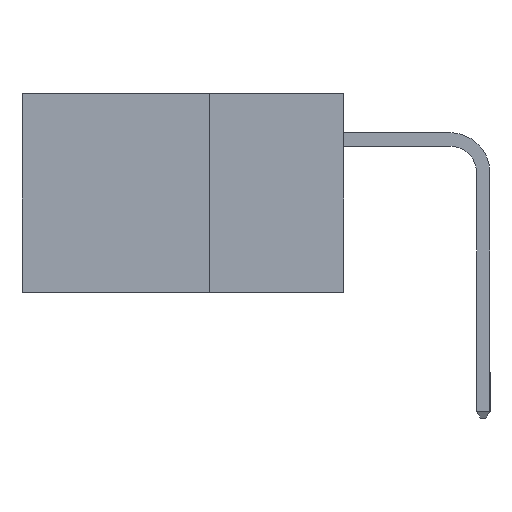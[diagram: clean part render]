
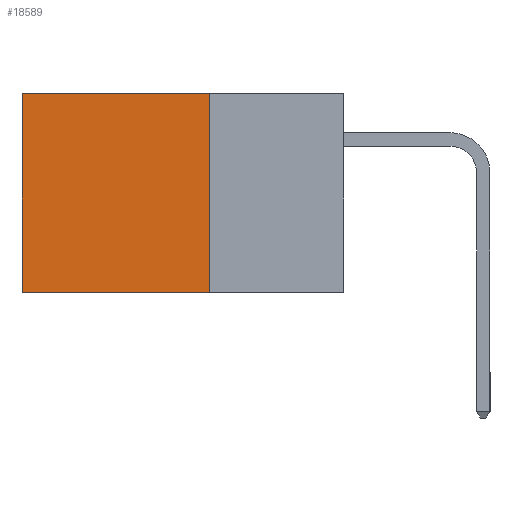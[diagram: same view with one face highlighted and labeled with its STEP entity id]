
A CAD part, left-side view. The second image highlights one B-rep face of the part: STEP entity #18589.
In plain terms, the highlighted planar face has unit normal (-1, 0, 0).
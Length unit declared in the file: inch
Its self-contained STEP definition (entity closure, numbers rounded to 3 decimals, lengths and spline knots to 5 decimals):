
#692 = DIRECTION ( 'NONE',  ( 1., 0., 0. ) ) ;
#1110 = VECTOR ( 'NONE', #4882, 39.37008 ) ;
#3337 = EDGE_LOOP ( 'NONE', ( #21907, #8122, #11441, #19299 ) ) ;
#3561 = EDGE_CURVE ( 'NONE', #12303, #6107, #20662, .T. ) ;
#4045 = CARTESIAN_POINT ( 'NONE',  ( 0.298, 0.25, -0.37 ) ) ;
#4882 = DIRECTION ( 'NONE',  ( 0., 0., -1. ) ) ;
#5588 = VECTOR ( 'NONE', #7385, 39.37008 ) ;
#5872 = AXIS2_PLACEMENT_3D ( 'NONE', #7417, #692, #7344 ) ;
#6041 = DIRECTION ( 'NONE',  ( 0., 1., 0. ) ) ;
#6107 = VERTEX_POINT ( 'NONE', #12417 ) ;
#6580 = VERTEX_POINT ( 'NONE', #14096 ) ;
#6591 = CARTESIAN_POINT ( 'NONE',  ( 0.298, 0.6, 0. ) ) ;
#7272 = FACE_OUTER_BOUND ( 'NONE', #3337, .T. ) ;
#7344 = DIRECTION ( 'NONE',  ( 0., 0., -1. ) ) ;
#7385 = DIRECTION ( 'NONE',  ( 0., 1., 0. ) ) ;
#7417 = CARTESIAN_POINT ( 'NONE',  ( 0.298, 0.25, 0. ) ) ;
#8122 = ORIENTED_EDGE ( 'NONE', *, *, #16086, .F. ) ;
#10761 = EDGE_CURVE ( 'NONE', #16242, #6580, #15560, .T. ) ;
#11339 = DIRECTION ( 'NONE',  ( 0., 0., -1. ) ) ;
#11441 = ORIENTED_EDGE ( 'NONE', *, *, #3561, .F. ) ;
#12303 = VERTEX_POINT ( 'NONE', #14629 ) ;
#12417 = CARTESIAN_POINT ( 'NONE',  ( 0.298, 0.25, -0.37 ) ) ;
#12716 = PLANE ( 'NONE',  #5872 ) ;
#13416 = CARTESIAN_POINT ( 'NONE',  ( 0.298, 0.6, 0. ) ) ;
#14096 = CARTESIAN_POINT ( 'NONE',  ( 0.298, 0.6, -0.37 ) ) ;
#14629 = CARTESIAN_POINT ( 'NONE',  ( 0.298, 0.25, 0. ) ) ;
#14650 = CARTESIAN_POINT ( 'NONE',  ( 0.298, 0.25, 0. ) ) ;
#15560 = LINE ( 'NONE', #6591, #1110 ) ;
#16086 = EDGE_CURVE ( 'NONE', #6107, #6580, #17613, .T. ) ;
#16242 = VERTEX_POINT ( 'NONE', #13416 ) ;
#16528 = VECTOR ( 'NONE', #6041, 39.37008 ) ;
#16706 = VECTOR ( 'NONE', #11339, 39.37008 ) ;
#17613 = LINE ( 'NONE', #4045, #16528 ) ;
#17620 = LINE ( 'NONE', #20652, #5588 ) ;
#18589 = ADVANCED_FACE ( 'NONE', ( #7272 ), #12716, .F. ) ;
#19299 = ORIENTED_EDGE ( 'NONE', *, *, #20382, .T. ) ;
#20382 = EDGE_CURVE ( 'NONE', #12303, #16242, #17620, .T. ) ;
#20652 = CARTESIAN_POINT ( 'NONE',  ( 0.298, 0.25, 0. ) ) ;
#20662 = LINE ( 'NONE', #14650, #16706 ) ;
#21907 = ORIENTED_EDGE ( 'NONE', *, *, #10761, .T. ) ;
